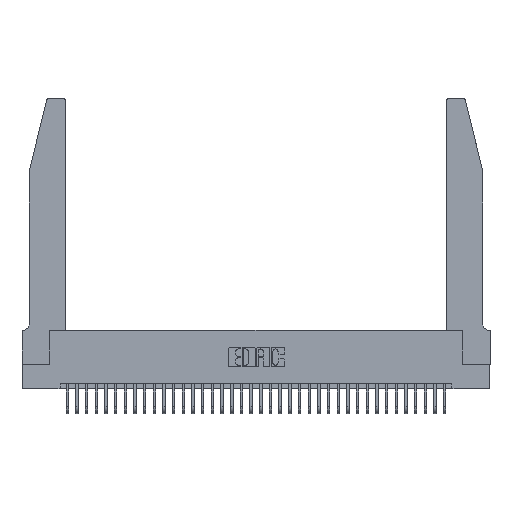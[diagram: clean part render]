
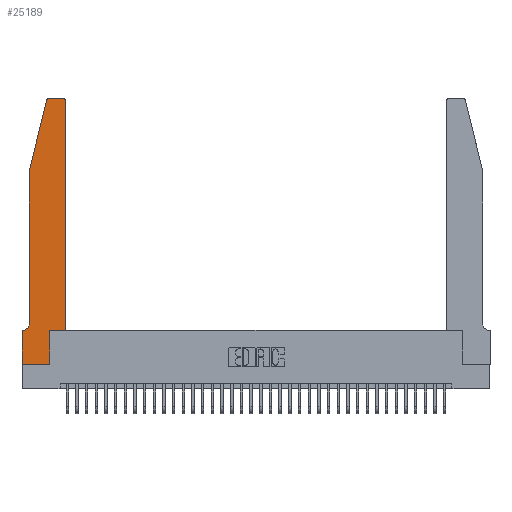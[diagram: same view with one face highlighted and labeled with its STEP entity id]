
A CAD part, top view. The second image highlights one B-rep face of the part: STEP entity #25189.
In plain terms, the highlighted planar face has unit normal (0, 0, 1).
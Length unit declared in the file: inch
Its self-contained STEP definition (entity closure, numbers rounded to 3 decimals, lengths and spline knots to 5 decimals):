
#249 = CARTESIAN_POINT ( 'NONE',  ( 0.2865, 0.35, 0.37 ) ) ;
#327 = VECTOR ( 'NONE', #24415, 39.37008 ) ;
#337 = CARTESIAN_POINT ( 'NONE',  ( 0.0755, 2., 0.37 ) ) ;
#344 = VERTEX_POINT ( 'NONE', #3460 ) ;
#419 = CARTESIAN_POINT ( 'NONE',  ( 0.4505, 0.35, 0.37 ) ) ;
#479 = DIRECTION ( 'NONE',  ( 0., 1., 0. ) ) ;
#527 = VERTEX_POINT ( 'NONE', #33215 ) ;
#1035 = DIRECTION ( 'NONE',  ( -0.239, -0.971, 0. ) ) ;
#1160 = EDGE_CURVE ( 'NONE', #14869, #28456, #2783, .T. ) ;
#1543 = EDGE_CURVE ( 'NONE', #35000, #19814, #21283, .T. ) ;
#1670 = LINE ( 'NONE', #15946, #24352 ) ;
#1689 = LINE ( 'NONE', #249, #32036 ) ;
#2228 = ORIENTED_EDGE ( 'NONE', *, *, #3120, .T. ) ;
#2478 = CARTESIAN_POINT ( 'NONE',  ( 0.4205, 2.72, 0.37 ) ) ;
#2783 = LINE ( 'NONE', #12464, #10784 ) ;
#3120 = EDGE_CURVE ( 'NONE', #19814, #17005, #1670, .T. ) ;
#3460 = CARTESIAN_POINT ( 'NONE',  ( 0.4205, 2.75, 0.37 ) ) ;
#3523 = DIRECTION ( 'NONE',  ( 1., 0., 0. ) ) ;
#3608 = VERTEX_POINT ( 'NONE', #32687 ) ;
#5551 = DIRECTION ( 'NONE',  ( 1., 0., 0. ) ) ;
#5913 = CARTESIAN_POINT ( 'NONE',  ( 0.0055, 0.42, 0.37 ) ) ;
#6084 = VECTOR ( 'NONE', #26836, 39.37008 ) ;
#7505 = ORIENTED_EDGE ( 'NONE', *, *, #25265, .T. ) ;
#7878 = AXIS2_PLACEMENT_3D ( 'NONE', #5913, #26445, #8912 ) ;
#8422 = DIRECTION ( 'NONE',  ( 0., 0., 1. ) ) ;
#8484 = EDGE_CURVE ( 'NONE', #28456, #344, #31211, .T. ) ;
#8828 = CARTESIAN_POINT ( 'NONE',  ( 0.2605, 2.75, 0.37 ) ) ;
#8912 = DIRECTION ( 'NONE',  ( -1., 0., 0. ) ) ;
#9338 = CARTESIAN_POINT ( 'NONE',  ( 0., 0., 0.37 ) ) ;
#9402 = EDGE_CURVE ( 'NONE', #30931, #35122, #1689, .T. ) ;
#9532 = DIRECTION ( 'NONE',  ( 0., 1., 0. ) ) ;
#9663 = CARTESIAN_POINT ( 'NONE',  ( 0.0055, 0.35, 0.37 ) ) ;
#10435 = CARTESIAN_POINT ( 'NONE',  ( 0.2865, 0., 0.37 ) ) ;
#10784 = VECTOR ( 'NONE', #479, 39.37008 ) ;
#10820 = CARTESIAN_POINT ( 'NONE',  ( 0.0755, 2., 0.37 ) ) ;
#11487 = AXIS2_PLACEMENT_3D ( 'NONE', #17394, #37641, #20273 ) ;
#12123 = VECTOR ( 'NONE', #3523, 39.37008 ) ;
#12464 = CARTESIAN_POINT ( 'NONE',  ( 0.4505, 0.35, 0.37 ) ) ;
#12925 = AXIS2_PLACEMENT_3D ( 'NONE', #2478, #23167, #5551 ) ;
#13995 = CARTESIAN_POINT ( 'NONE',  ( 0.284, 2.75, 0.37 ) ) ;
#14415 = LINE ( 'NONE', #10820, #28930 ) ;
#14869 = VERTEX_POINT ( 'NONE', #37598 ) ;
#15029 = DIRECTION ( 'NONE',  ( 0., -1., 0. ) ) ;
#15111 = ORIENTED_EDGE ( 'NONE', *, *, #25392, .T. ) ;
#15369 = ORIENTED_EDGE ( 'NONE', *, *, #19905, .T. ) ;
#15798 = ORIENTED_EDGE ( 'NONE', *, *, #35816, .T. ) ;
#15799 = CARTESIAN_POINT ( 'NONE',  ( 0.4505, 2.72, 0.37 ) ) ;
#15946 = CARTESIAN_POINT ( 'NONE',  ( 0.0755, 2., 0.37 ) ) ;
#17005 = VERTEX_POINT ( 'NONE', #337 ) ;
#17394 = CARTESIAN_POINT ( 'NONE',  ( 0., 0.35, 0.37 ) ) ;
#17442 = VECTOR ( 'NONE', #15029, 39.37008 ) ;
#17705 = CIRCLE ( 'NONE', #7878, 0.07 ) ;
#18263 = VERTEX_POINT ( 'NONE', #9663 ) ;
#18273 = ORIENTED_EDGE ( 'NONE', *, *, #35945, .T. ) ;
#19814 = VERTEX_POINT ( 'NONE', #33716 ) ;
#19905 = EDGE_CURVE ( 'NONE', #17005, #29285, #14415, .T. ) ;
#20273 = DIRECTION ( 'NONE',  ( 1., 0., 0. ) ) ;
#21283 = CIRCLE ( 'NONE', #26904, 0.03 ) ;
#21894 = ORIENTED_EDGE ( 'NONE', *, *, #36077, .T. ) ;
#23167 = DIRECTION ( 'NONE',  ( 0., 0., 1. ) ) ;
#23241 = ORIENTED_EDGE ( 'NONE', *, *, #1543, .T. ) ;
#24352 = VECTOR ( 'NONE', #1035, 39.37008 ) ;
#24415 = DIRECTION ( 'NONE',  ( -1., 0., 0. ) ) ;
#25114 = ORIENTED_EDGE ( 'NONE', *, *, #9402, .T. ) ;
#25141 = LINE ( 'NONE', #32389, #17442 ) ;
#25189 = ADVANCED_FACE ( 'NONE', ( #26324 ), #28865, .T. ) ;
#25265 = EDGE_CURVE ( 'NONE', #344, #35000, #25418, .T. ) ;
#25392 = EDGE_CURVE ( 'NONE', #527, #30931, #28536, .T. ) ;
#25418 = LINE ( 'NONE', #8828, #31280 ) ;
#25973 = CARTESIAN_POINT ( 'NONE',  ( 0.284, 2.72, 0.37 ) ) ;
#26324 = FACE_OUTER_BOUND ( 'NONE', #33024, .T. ) ;
#26368 = DIRECTION ( 'NONE',  ( -1., 0., 0. ) ) ;
#26445 = DIRECTION ( 'NONE',  ( 0., 0., -1. ) ) ;
#26836 = DIRECTION ( 'NONE',  ( 1., 0., 0. ) ) ;
#26904 = AXIS2_PLACEMENT_3D ( 'NONE', #25973, #8422, #28841 ) ;
#28256 = DIRECTION ( 'NONE',  ( 0., -1., 0. ) ) ;
#28456 = VERTEX_POINT ( 'NONE', #15799 ) ;
#28536 = LINE ( 'NONE', #9338, #6084 ) ;
#28841 = DIRECTION ( 'NONE',  ( 1., 0., 0. ) ) ;
#28865 = PLANE ( 'NONE',  #11487 ) ;
#28930 = VECTOR ( 'NONE', #28256, 39.37008 ) ;
#28962 = CARTESIAN_POINT ( 'NONE',  ( 0.2865, 0.35, 0.37 ) ) ;
#29285 = VERTEX_POINT ( 'NONE', #31441 ) ;
#30778 = LINE ( 'NONE', #33239, #327 ) ;
#30931 = VERTEX_POINT ( 'NONE', #10435 ) ;
#31211 = CIRCLE ( 'NONE', #12925, 0.03 ) ;
#31280 = VECTOR ( 'NONE', #26368, 39.37008 ) ;
#31441 = CARTESIAN_POINT ( 'NONE',  ( 0.0755, 0.42, 0.37 ) ) ;
#32036 = VECTOR ( 'NONE', #9532, 39.37008 ) ;
#32389 = CARTESIAN_POINT ( 'NONE',  ( 0., 0., 0.37 ) ) ;
#32687 = CARTESIAN_POINT ( 'NONE',  ( 0., 0.35, 0.37 ) ) ;
#33024 = EDGE_LOOP ( 'NONE', ( #7505, #23241, #2228, #15369, #15798, #21894, #33347, #15111, #25114, #18273, #37791, #34854 ) ) ;
#33215 = CARTESIAN_POINT ( 'NONE',  ( 0., 0., 0.37 ) ) ;
#33239 = CARTESIAN_POINT ( 'NONE',  ( 0.0755, 0.35, 0.37 ) ) ;
#33259 = EDGE_CURVE ( 'NONE', #3608, #527, #25141, .T. ) ;
#33347 = ORIENTED_EDGE ( 'NONE', *, *, #33259, .T. ) ;
#33716 = CARTESIAN_POINT ( 'NONE',  ( 0.25487, 2.72718, 0.37 ) ) ;
#34854 = ORIENTED_EDGE ( 'NONE', *, *, #8484, .T. ) ;
#35000 = VERTEX_POINT ( 'NONE', #13995 ) ;
#35122 = VERTEX_POINT ( 'NONE', #28962 ) ;
#35355 = LINE ( 'NONE', #419, #12123 ) ;
#35816 = EDGE_CURVE ( 'NONE', #29285, #18263, #17705, .T. ) ;
#35945 = EDGE_CURVE ( 'NONE', #35122, #14869, #35355, .T. ) ;
#36077 = EDGE_CURVE ( 'NONE', #18263, #3608, #30778, .T. ) ;
#37598 = CARTESIAN_POINT ( 'NONE',  ( 0.4505, 0.35, 0.37 ) ) ;
#37641 = DIRECTION ( 'NONE',  ( 0., 0., 1. ) ) ;
#37791 = ORIENTED_EDGE ( 'NONE', *, *, #1160, .T. ) ;
